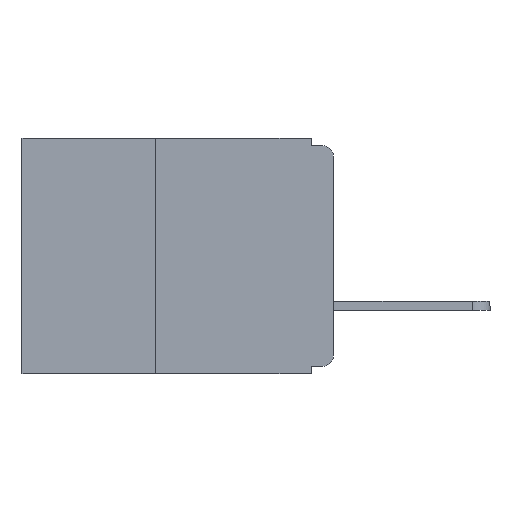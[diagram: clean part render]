
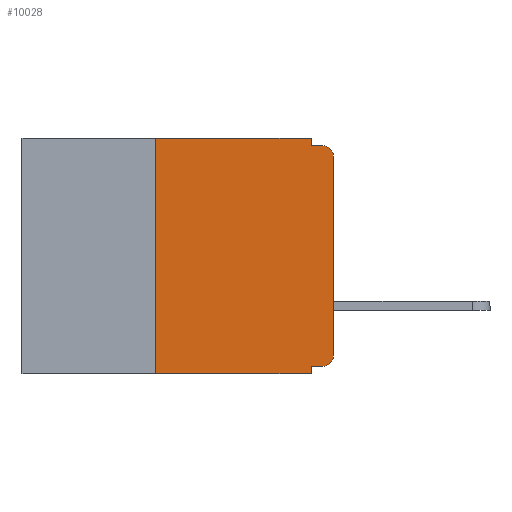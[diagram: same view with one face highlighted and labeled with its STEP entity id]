
A CAD part, left-side view. The second image highlights one B-rep face of the part: STEP entity #10028.
In plain terms, the highlighted planar face has unit normal (-1, 0, 0).
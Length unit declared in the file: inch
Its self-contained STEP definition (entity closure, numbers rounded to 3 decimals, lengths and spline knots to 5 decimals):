
#6 = DIRECTION ( 'NONE',  ( -1., 0., 0. ) ) ;
#227 = CARTESIAN_POINT ( 'NONE',  ( 0., 0.015, -0.025 ) ) ;
#249 = LINE ( 'NONE', #24679, #28201 ) ;
#1717 = EDGE_CURVE ( 'NONE', #3015, #15254, #26719, .T. ) ;
#1928 = EDGE_CURVE ( 'NONE', #28345, #29555, #34283, .T. ) ;
#2233 = AXIS2_PLACEMENT_3D ( 'NONE', #33083, #12173, #30974 ) ;
#3015 = VERTEX_POINT ( 'NONE', #6258 ) ;
#3453 = ORIENTED_EDGE ( 'NONE', *, *, #21794, .F. ) ;
#4101 = ORIENTED_EDGE ( 'NONE', *, *, #6919, .T. ) ;
#4958 = VECTOR ( 'NONE', #17626, 39.37008 ) ;
#5511 = CARTESIAN_POINT ( 'NONE',  ( 0., 0., 0. ) ) ;
#5557 = EDGE_CURVE ( 'NONE', #28783, #3015, #31090, .T. ) ;
#5867 = LINE ( 'NONE', #24908, #26491 ) ;
#6227 = CARTESIAN_POINT ( 'NONE',  ( 0., 0.031, 0. ) ) ;
#6258 = CARTESIAN_POINT ( 'NONE',  ( 0., 0.25, 0. ) ) ;
#6425 = ORIENTED_EDGE ( 'NONE', *, *, #31539, .T. ) ;
#6676 = DIRECTION ( 'NONE',  ( 0., 0., -1. ) ) ;
#6763 = CARTESIAN_POINT ( 'NONE',  ( 0., 0.25, -0.33 ) ) ;
#6797 = AXIS2_PLACEMENT_3D ( 'NONE', #227, #6, #6676 ) ;
#6919 = EDGE_CURVE ( 'NONE', #19758, #8962, #7839, .T. ) ;
#6939 = CARTESIAN_POINT ( 'NONE',  ( 0., 0., -0.305 ) ) ;
#7839 = CIRCLE ( 'NONE', #12210, 0.015 ) ;
#8241 = DIRECTION ( 'NONE',  ( 0., 0., 1. ) ) ;
#8599 = VERTEX_POINT ( 'NONE', #24239 ) ;
#8933 = DIRECTION ( 'NONE',  ( 0., 0., -1. ) ) ;
#8962 = VERTEX_POINT ( 'NONE', #6939 ) ;
#9168 = ORIENTED_EDGE ( 'NONE', *, *, #5557, .F. ) ;
#9317 = ORIENTED_EDGE ( 'NONE', *, *, #1928, .T. ) ;
#9876 = ORIENTED_EDGE ( 'NONE', *, *, #1717, .F. ) ;
#10028 = ADVANCED_FACE ( 'NONE', ( #13544 ), #28281, .F. ) ;
#10229 = CARTESIAN_POINT ( 'NONE',  ( 0., 0.015, -0.305 ) ) ;
#11733 = VERTEX_POINT ( 'NONE', #17816 ) ;
#12173 = DIRECTION ( 'NONE',  ( 1., 0., 0. ) ) ;
#12210 = AXIS2_PLACEMENT_3D ( 'NONE', #10229, #29032, #12930 ) ;
#12569 = ORIENTED_EDGE ( 'NONE', *, *, #15081, .F. ) ;
#12756 = EDGE_CURVE ( 'NONE', #15254, #11733, #26213, .T. ) ;
#12930 = DIRECTION ( 'NONE',  ( 0., 0., -1. ) ) ;
#13053 = ORIENTED_EDGE ( 'NONE', *, *, #31589, .F. ) ;
#13450 = DIRECTION ( 'NONE',  ( 0., -1., 0. ) ) ;
#13544 = FACE_OUTER_BOUND ( 'NONE', #34981, .T. ) ;
#14197 = EDGE_CURVE ( 'NONE', #8962, #28345, #28222, .T. ) ;
#15081 = EDGE_CURVE ( 'NONE', #11733, #29555, #28153, .T. ) ;
#15254 = VERTEX_POINT ( 'NONE', #31892 ) ;
#15417 = CARTESIAN_POINT ( 'NONE',  ( 0., 0.437, 0. ) ) ;
#16675 = DIRECTION ( 'NONE',  ( 0., -1., 0. ) ) ;
#17045 = CARTESIAN_POINT ( 'NONE',  ( 0., 0., -0.025 ) ) ;
#17566 = CARTESIAN_POINT ( 'NONE',  ( 0., 0., -0.01 ) ) ;
#17626 = DIRECTION ( 'NONE',  ( 0., 1., 0. ) ) ;
#17816 = CARTESIAN_POINT ( 'NONE',  ( 0., 0.031, -0.01 ) ) ;
#18021 = CARTESIAN_POINT ( 'NONE',  ( 0., 0.031, -0.32 ) ) ;
#18432 = LINE ( 'NONE', #31055, #4958 ) ;
#19573 = VECTOR ( 'NONE', #13450, 39.37008 ) ;
#19758 = VERTEX_POINT ( 'NONE', #24360 ) ;
#19911 = VECTOR ( 'NONE', #8933, 39.37008 ) ;
#20206 = VECTOR ( 'NONE', #8241, 39.37008 ) ;
#21794 = EDGE_CURVE ( 'NONE', #19758, #32498, #18432, .T. ) ;
#22391 = CARTESIAN_POINT ( 'NONE',  ( 0., 0.015, -0.01 ) ) ;
#24239 = CARTESIAN_POINT ( 'NONE',  ( 0., 0.031, -0.33 ) ) ;
#24360 = CARTESIAN_POINT ( 'NONE',  ( 0., 0.015, -0.32 ) ) ;
#24679 = CARTESIAN_POINT ( 'NONE',  ( 0., 0.437, -0.33 ) ) ;
#24775 = VECTOR ( 'NONE', #25585, 39.37008 ) ;
#24908 = CARTESIAN_POINT ( 'NONE',  ( 0., 0.031, -0.33 ) ) ;
#25585 = DIRECTION ( 'NONE',  ( 0., 0., 1. ) ) ;
#26213 = LINE ( 'NONE', #6227, #19911 ) ;
#26491 = VECTOR ( 'NONE', #27625, 39.37008 ) ;
#26719 = LINE ( 'NONE', #15417, #19573 ) ;
#27148 = CARTESIAN_POINT ( 'NONE',  ( 0., 0.25, -0.33 ) ) ;
#27625 = DIRECTION ( 'NONE',  ( 0., 0., -1. ) ) ;
#28153 = LINE ( 'NONE', #17566, #33612 ) ;
#28201 = VECTOR ( 'NONE', #16675, 39.37008 ) ;
#28222 = LINE ( 'NONE', #5511, #20206 ) ;
#28281 = PLANE ( 'NONE',  #2233 ) ;
#28345 = VERTEX_POINT ( 'NONE', #17045 ) ;
#28783 = VERTEX_POINT ( 'NONE', #27148 ) ;
#29032 = DIRECTION ( 'NONE',  ( -1., 0., 0. ) ) ;
#29555 = VERTEX_POINT ( 'NONE', #22391 ) ;
#30092 = ORIENTED_EDGE ( 'NONE', *, *, #12756, .F. ) ;
#30974 = DIRECTION ( 'NONE',  ( 0., 0., -1. ) ) ;
#31055 = CARTESIAN_POINT ( 'NONE',  ( 0., 0., -0.32 ) ) ;
#31090 = LINE ( 'NONE', #6763, #24775 ) ;
#31539 = EDGE_CURVE ( 'NONE', #28783, #8599, #249, .T. ) ;
#31589 = EDGE_CURVE ( 'NONE', #32498, #8599, #5867, .T. ) ;
#31892 = CARTESIAN_POINT ( 'NONE',  ( 0., 0.031, 0. ) ) ;
#32498 = VERTEX_POINT ( 'NONE', #18021 ) ;
#33083 = CARTESIAN_POINT ( 'NONE',  ( 0., 0.437, 0. ) ) ;
#33612 = VECTOR ( 'NONE', #33698, 39.37008 ) ;
#33652 = ORIENTED_EDGE ( 'NONE', *, *, #14197, .T. ) ;
#33698 = DIRECTION ( 'NONE',  ( 0., -1., 0. ) ) ;
#34283 = CIRCLE ( 'NONE', #6797, 0.015 ) ;
#34981 = EDGE_LOOP ( 'NONE', ( #33652, #9317, #12569, #30092, #9876, #9168, #6425, #13053, #3453, #4101 ) ) ;
